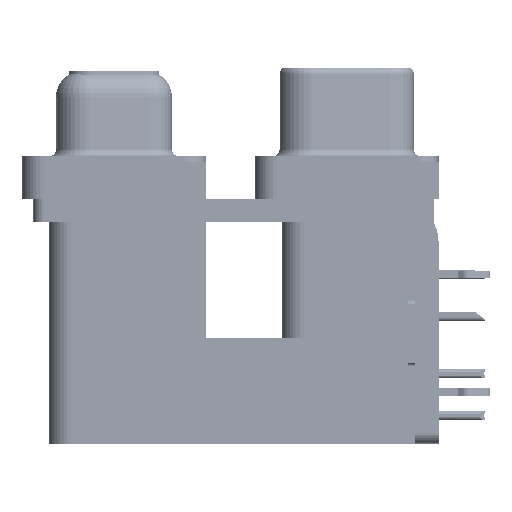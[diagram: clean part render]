
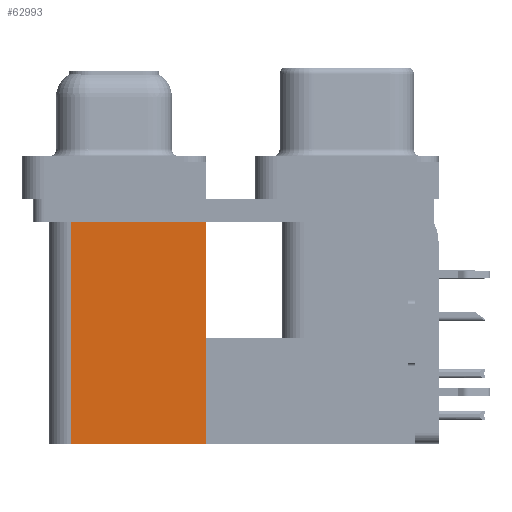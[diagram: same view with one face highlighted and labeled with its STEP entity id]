
A CAD part, left-side view. The second image highlights one B-rep face of the part: STEP entity #62993.
In plain terms, the highlighted planar face has unit normal (-1, 0, 0).
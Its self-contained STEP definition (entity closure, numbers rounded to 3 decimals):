
#1033 = CARTESIAN_POINT ( 'NONE',  ( 3.79, 9.6, -19.2 ) ) ;
#1392 = LINE ( 'NONE', #22333, #16018 ) ;
#3395 = CARTESIAN_POINT ( 'NONE',  ( 3.79, 9.6, -19.2 ) ) ;
#3763 = CARTESIAN_POINT ( 'NONE',  ( 3.79, 18.8, -2.5 ) ) ;
#6647 = VECTOR ( 'NONE', #30731, 1000. ) ;
#7204 = VERTEX_POINT ( 'NONE', #46079 ) ;
#8553 = LINE ( 'NONE', #3395, #46257 ) ;
#9776 = LINE ( 'NONE', #14594, #6647 ) ;
#14594 = CARTESIAN_POINT ( 'NONE',  ( 3.79, 9.6, -19.2 ) ) ;
#16018 = VECTOR ( 'NONE', #52939, 1000. ) ;
#16324 = EDGE_CURVE ( 'NONE', #7204, #28181, #59393, .T. ) ;
#22333 = CARTESIAN_POINT ( 'NONE',  ( 3.79, 9.6, -2.5 ) ) ;
#24030 = DIRECTION ( 'NONE',  ( 1., 0., 0. ) ) ;
#25450 = VECTOR ( 'NONE', #54230, 1000. ) ;
#26811 = EDGE_CURVE ( 'NONE', #62327, #28181, #1392, .T. ) ;
#28181 = VERTEX_POINT ( 'NONE', #3763 ) ;
#29194 = PLANE ( 'NONE',  #30509 ) ;
#29521 = DIRECTION ( 'NONE',  ( 0., 0., 1. ) ) ;
#29524 = FACE_OUTER_BOUND ( 'NONE', #57858, .T. ) ;
#30509 = AXIS2_PLACEMENT_3D ( 'NONE', #50145, #24030, #50475 ) ;
#30731 = DIRECTION ( 'NONE',  ( 0., 1., 0. ) ) ;
#32608 = CARTESIAN_POINT ( 'NONE',  ( 3.79, 18.8, -19.2 ) ) ;
#35476 = EDGE_CURVE ( 'NONE', #46818, #7204, #9776, .T. ) ;
#42288 = ORIENTED_EDGE ( 'NONE', *, *, #66295, .T. ) ;
#46079 = CARTESIAN_POINT ( 'NONE',  ( 3.79, 18.8, -19.2 ) ) ;
#46257 = VECTOR ( 'NONE', #29521, 1000. ) ;
#46818 = VERTEX_POINT ( 'NONE', #1033 ) ;
#47184 = CARTESIAN_POINT ( 'NONE',  ( 3.79, 9.6, -2.5 ) ) ;
#50145 = CARTESIAN_POINT ( 'NONE',  ( 3.79, 9.6, -19.2 ) ) ;
#50475 = DIRECTION ( 'NONE',  ( 0., 1., 0. ) ) ;
#52721 = ORIENTED_EDGE ( 'NONE', *, *, #35476, .F. ) ;
#52939 = DIRECTION ( 'NONE',  ( 0., 1., 0. ) ) ;
#54230 = DIRECTION ( 'NONE',  ( 0., 0., 1. ) ) ;
#57858 = EDGE_LOOP ( 'NONE', ( #65843, #67248, #52721, #42288 ) ) ;
#59393 = LINE ( 'NONE', #32608, #25450 ) ;
#62327 = VERTEX_POINT ( 'NONE', #47184 ) ;
#62993 = ADVANCED_FACE ( 'NONE', ( #29524 ), #29194, .F. ) ;
#65843 = ORIENTED_EDGE ( 'NONE', *, *, #26811, .T. ) ;
#66295 = EDGE_CURVE ( 'NONE', #46818, #62327, #8553, .T. ) ;
#67248 = ORIENTED_EDGE ( 'NONE', *, *, #16324, .F. ) ;
